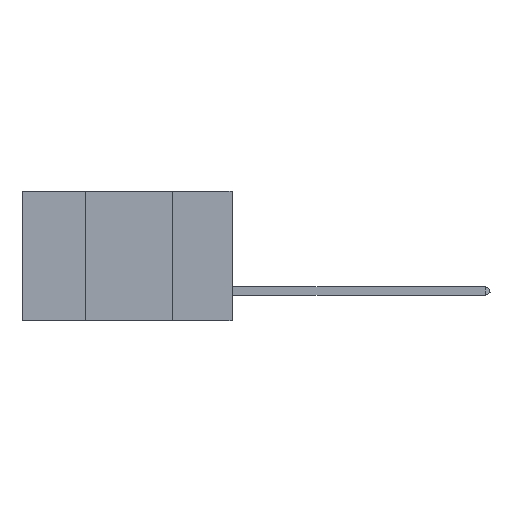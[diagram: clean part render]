
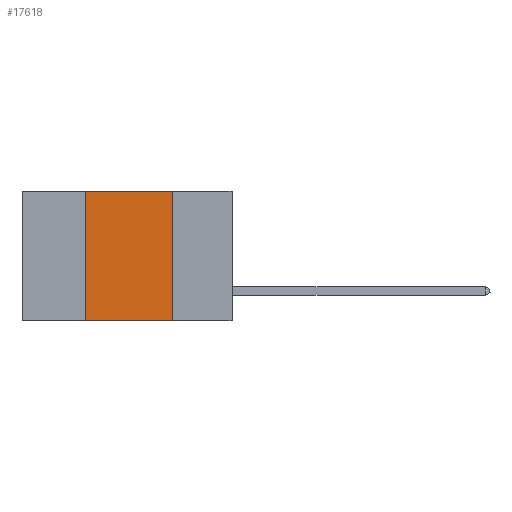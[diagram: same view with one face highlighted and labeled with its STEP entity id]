
A CAD part, left-side view. The second image highlights one B-rep face of the part: STEP entity #17618.
In plain terms, the highlighted planar face has unit normal (-1, 0, 0).
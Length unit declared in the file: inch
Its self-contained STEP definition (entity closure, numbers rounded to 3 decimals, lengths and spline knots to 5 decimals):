
#2454 = DIRECTION ( 'NONE',  ( 0., -1., 0. ) ) ;
#2523 = VECTOR ( 'NONE', #2454, 39.37008 ) ;
#2781 = LINE ( 'NONE', #25417, #30321 ) ;
#3811 = DIRECTION ( 'NONE',  ( 0., -1., 0. ) ) ;
#3983 = VERTEX_POINT ( 'NONE', #38807 ) ;
#4551 = CARTESIAN_POINT ( 'NONE',  ( 0., 0.17, -0.37 ) ) ;
#5003 = EDGE_LOOP ( 'NONE', ( #33518, #43424, #37874, #16635 ) ) ;
#5231 = FACE_OUTER_BOUND ( 'NONE', #5003, .T. ) ;
#8386 = CARTESIAN_POINT ( 'NONE',  ( 0., 0.17, 0. ) ) ;
#9264 = CARTESIAN_POINT ( 'NONE',  ( 0., 0.42, 0. ) ) ;
#11860 = VERTEX_POINT ( 'NONE', #4551 ) ;
#13149 = CARTESIAN_POINT ( 'NONE',  ( 0., 0.6, 0. ) ) ;
#13420 = VECTOR ( 'NONE', #3811, 39.37008 ) ;
#15587 = VECTOR ( 'NONE', #21258, 39.37008 ) ;
#16635 = ORIENTED_EDGE ( 'NONE', *, *, #34432, .T. ) ;
#16916 = EDGE_CURVE ( 'NONE', #32627, #28308, #25585, .T. ) ;
#17618 = ADVANCED_FACE ( 'NONE', ( #5231 ), #21422, .F. ) ;
#19839 = EDGE_CURVE ( 'NONE', #3983, #32627, #2781, .T. ) ;
#21258 = DIRECTION ( 'NONE',  ( 0., 0., -1. ) ) ;
#21422 = PLANE ( 'NONE',  #30293 ) ;
#25417 = CARTESIAN_POINT ( 'NONE',  ( 0., 0.42, 0. ) ) ;
#25585 = LINE ( 'NONE', #13149, #2523 ) ;
#26900 = LINE ( 'NONE', #29104, #13420 ) ;
#28308 = VERTEX_POINT ( 'NONE', #8386 ) ;
#28856 = DIRECTION ( 'NONE',  ( 0., 0., 1. ) ) ;
#29059 = LINE ( 'NONE', #35639, #15587 ) ;
#29104 = CARTESIAN_POINT ( 'NONE',  ( 0., 0.6, -0.37 ) ) ;
#30293 = AXIS2_PLACEMENT_3D ( 'NONE', #35176, #43010, #32057 ) ;
#30321 = VECTOR ( 'NONE', #28856, 39.37008 ) ;
#32057 = DIRECTION ( 'NONE',  ( 0., 0., -1. ) ) ;
#32203 = EDGE_CURVE ( 'NONE', #28308, #11860, #29059, .T. ) ;
#32627 = VERTEX_POINT ( 'NONE', #9264 ) ;
#33518 = ORIENTED_EDGE ( 'NONE', *, *, #32203, .F. ) ;
#34432 = EDGE_CURVE ( 'NONE', #3983, #11860, #26900, .T. ) ;
#35176 = CARTESIAN_POINT ( 'NONE',  ( 0., 0.6, 0. ) ) ;
#35639 = CARTESIAN_POINT ( 'NONE',  ( 0., 0.17, 0. ) ) ;
#37874 = ORIENTED_EDGE ( 'NONE', *, *, #19839, .F. ) ;
#38807 = CARTESIAN_POINT ( 'NONE',  ( 0., 0.42, -0.37 ) ) ;
#43010 = DIRECTION ( 'NONE',  ( 1., 0., 0. ) ) ;
#43424 = ORIENTED_EDGE ( 'NONE', *, *, #16916, .F. ) ;
